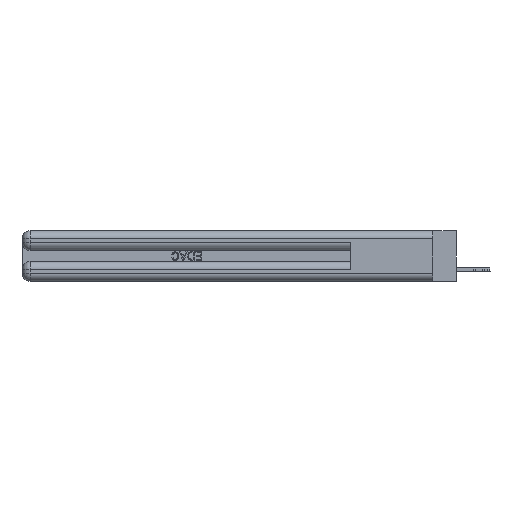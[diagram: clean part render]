
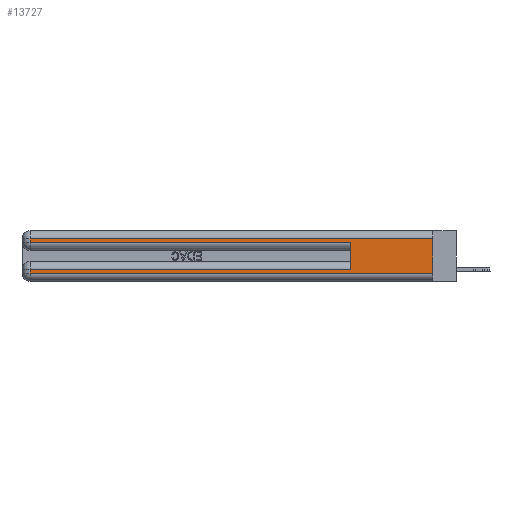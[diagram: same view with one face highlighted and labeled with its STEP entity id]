
A CAD part, left-side view. The second image highlights one B-rep face of the part: STEP entity #13727.
In plain terms, the highlighted planar face has unit normal (-1, 0, 0).
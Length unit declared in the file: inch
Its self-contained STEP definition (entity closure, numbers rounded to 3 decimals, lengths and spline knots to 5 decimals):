
#222 = FACE_OUTER_BOUND ( 'NONE', #21742, .T. ) ;
#477 = EDGE_CURVE ( 'NONE', #37483, #5347, #39453, .T. ) ;
#928 = LINE ( 'NONE', #38696, #26078 ) ;
#1338 = DIRECTION ( 'NONE',  ( 0., 0., -1. ) ) ;
#1611 = CARTESIAN_POINT ( 'NONE',  ( 0., 2.94, 0.31 ) ) ;
#1694 = DIRECTION ( 'NONE',  ( 0., 0., -1. ) ) ;
#2288 = ORIENTED_EDGE ( 'NONE', *, *, #11927, .T. ) ;
#2511 = CARTESIAN_POINT ( 'NONE',  ( 0., 2.94, 0.06 ) ) ;
#2580 = CARTESIAN_POINT ( 'NONE',  ( 0., 0., 0.06 ) ) ;
#2890 = CARTESIAN_POINT ( 'NONE',  ( 0., 0., 0.31 ) ) ;
#5048 = VERTEX_POINT ( 'NONE', #16108 ) ;
#5347 = VERTEX_POINT ( 'NONE', #22084 ) ;
#5360 = VERTEX_POINT ( 'NONE', #1611 ) ;
#6093 = AXIS2_PLACEMENT_3D ( 'NONE', #14399, #21559, #38300 ) ;
#7520 = EDGE_CURVE ( 'NONE', #5360, #5048, #30851, .T. ) ;
#9595 = VECTOR ( 'NONE', #19753, 39.37008 ) ;
#9938 = VERTEX_POINT ( 'NONE', #2511 ) ;
#10257 = EDGE_CURVE ( 'NONE', #37483, #38684, #17598, .T. ) ;
#10533 = CARTESIAN_POINT ( 'NONE',  ( 0., 0.6, 0.145 ) ) ;
#10729 = CARTESIAN_POINT ( 'NONE',  ( 0., 2.94, 0.37 ) ) ;
#11927 = EDGE_CURVE ( 'NONE', #9938, #16178, #23281, .T. ) ;
#13623 = ORIENTED_EDGE ( 'NONE', *, *, #10257, .T. ) ;
#13727 = ADVANCED_FACE ( 'NONE', ( #222 ), #38590, .F. ) ;
#13945 = DIRECTION ( 'NONE',  ( 0., -1., 0. ) ) ;
#14020 = DIRECTION ( 'NONE',  ( 0., 0., -1. ) ) ;
#14399 = CARTESIAN_POINT ( 'NONE',  ( 0., 0., 0.37 ) ) ;
#15369 = EDGE_CURVE ( 'NONE', #26529, #5360, #31142, .T. ) ;
#15465 = CARTESIAN_POINT ( 'NONE',  ( 0., 0., 0.37 ) ) ;
#16108 = CARTESIAN_POINT ( 'NONE',  ( 0., 2.94, 0.285 ) ) ;
#16178 = VERTEX_POINT ( 'NONE', #18599 ) ;
#17034 = CARTESIAN_POINT ( 'NONE',  ( 0., 0.6, 0.085 ) ) ;
#17226 = ORIENTED_EDGE ( 'NONE', *, *, #7520, .T. ) ;
#17433 = VECTOR ( 'NONE', #40208, 39.37008 ) ;
#17598 = LINE ( 'NONE', #19153, #9595 ) ;
#18599 = CARTESIAN_POINT ( 'NONE',  ( 0., 0., 0.06 ) ) ;
#19153 = CARTESIAN_POINT ( 'NONE',  ( 0., 0., 0.085 ) ) ;
#19717 = VECTOR ( 'NONE', #37461, 39.37008 ) ;
#19753 = DIRECTION ( 'NONE',  ( 0., 1., 0. ) ) ;
#20963 = VECTOR ( 'NONE', #33657, 39.37008 ) ;
#21559 = DIRECTION ( 'NONE',  ( 1., 0., 0. ) ) ;
#21742 = EDGE_LOOP ( 'NONE', ( #38424, #22887, #17226, #43830, #41695, #13623, #38655, #2288 ) ) ;
#22084 = CARTESIAN_POINT ( 'NONE',  ( 0., 0.6, 0.285 ) ) ;
#22127 = EDGE_CURVE ( 'NONE', #5048, #5347, #24336, .T. ) ;
#22887 = ORIENTED_EDGE ( 'NONE', *, *, #15369, .T. ) ;
#23281 = LINE ( 'NONE', #2580, #17433 ) ;
#23611 = EDGE_CURVE ( 'NONE', #26529, #16178, #26979, .T. ) ;
#24336 = LINE ( 'NONE', #27521, #27558 ) ;
#26078 = VECTOR ( 'NONE', #1338, 39.37008 ) ;
#26529 = VERTEX_POINT ( 'NONE', #31978 ) ;
#26979 = LINE ( 'NONE', #15465, #28537 ) ;
#27521 = CARTESIAN_POINT ( 'NONE',  ( 0., 0., 0.285 ) ) ;
#27558 = VECTOR ( 'NONE', #13945, 39.37008 ) ;
#28537 = VECTOR ( 'NONE', #1694, 39.37008 ) ;
#30851 = LINE ( 'NONE', #10729, #31335 ) ;
#31142 = LINE ( 'NONE', #2890, #20963 ) ;
#31335 = VECTOR ( 'NONE', #14020, 39.37008 ) ;
#31978 = CARTESIAN_POINT ( 'NONE',  ( 0., 0., 0.31 ) ) ;
#33657 = DIRECTION ( 'NONE',  ( 0., 1., 0. ) ) ;
#34106 = EDGE_CURVE ( 'NONE', #38684, #9938, #928, .T. ) ;
#37461 = DIRECTION ( 'NONE',  ( 0., 0., 1. ) ) ;
#37483 = VERTEX_POINT ( 'NONE', #17034 ) ;
#38300 = DIRECTION ( 'NONE',  ( 0., 0., -1. ) ) ;
#38424 = ORIENTED_EDGE ( 'NONE', *, *, #23611, .F. ) ;
#38590 = PLANE ( 'NONE',  #6093 ) ;
#38655 = ORIENTED_EDGE ( 'NONE', *, *, #34106, .T. ) ;
#38684 = VERTEX_POINT ( 'NONE', #40861 ) ;
#38696 = CARTESIAN_POINT ( 'NONE',  ( 0., 2.94, 0.37 ) ) ;
#39453 = LINE ( 'NONE', #10533, #19717 ) ;
#40208 = DIRECTION ( 'NONE',  ( 0., -1., 0. ) ) ;
#40861 = CARTESIAN_POINT ( 'NONE',  ( 0., 2.94, 0.085 ) ) ;
#41695 = ORIENTED_EDGE ( 'NONE', *, *, #477, .F. ) ;
#43830 = ORIENTED_EDGE ( 'NONE', *, *, #22127, .T. ) ;
